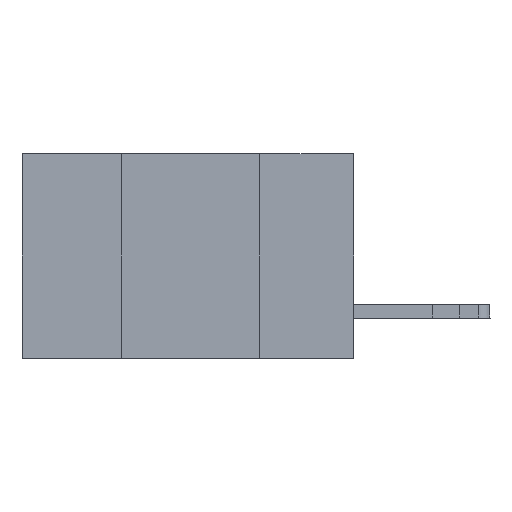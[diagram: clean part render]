
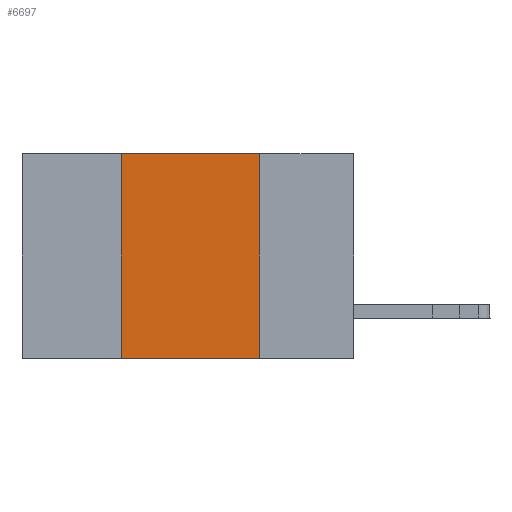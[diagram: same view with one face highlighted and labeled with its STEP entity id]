
A CAD part, left-side view. The second image highlights one B-rep face of the part: STEP entity #6697.
In plain terms, the highlighted planar face has unit normal (-1, 0, 0).
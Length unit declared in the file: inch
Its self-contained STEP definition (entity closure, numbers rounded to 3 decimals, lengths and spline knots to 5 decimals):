
#640 = PLANE ( 'NONE',  #17422 ) ;
#1142 = VERTEX_POINT ( 'NONE', #27740 ) ;
#1392 = LINE ( 'NONE', #13812, #27585 ) ;
#4769 = CARTESIAN_POINT ( 'NONE',  ( 0., 0.6, 0. ) ) ;
#6697 = ADVANCED_FACE ( 'NONE', ( #7841 ), #640, .F. ) ;
#7841 = FACE_OUTER_BOUND ( 'NONE', #24809, .T. ) ;
#8681 = EDGE_CURVE ( 'NONE', #14372, #1142, #14661, .T. ) ;
#9336 = CARTESIAN_POINT ( 'NONE',  ( 0., 0.17, 0. ) ) ;
#9477 = ORIENTED_EDGE ( 'NONE', *, *, #16613, .F. ) ;
#11644 = LINE ( 'NONE', #9336, #30288 ) ;
#12538 = EDGE_CURVE ( 'NONE', #13176, #19189, #24336, .T. ) ;
#13176 = VERTEX_POINT ( 'NONE', #31126 ) ;
#13812 = CARTESIAN_POINT ( 'NONE',  ( 0., 0.42, 0. ) ) ;
#14372 = VERTEX_POINT ( 'NONE', #31003 ) ;
#14661 = LINE ( 'NONE', #17255, #20536 ) ;
#16576 = DIRECTION ( 'NONE',  ( 0., 0., 1. ) ) ;
#16613 = EDGE_CURVE ( 'NONE', #14372, #13176, #1392, .T. ) ;
#16631 = CARTESIAN_POINT ( 'NONE',  ( 0., 0.17, 0. ) ) ;
#16641 = ORIENTED_EDGE ( 'NONE', *, *, #12538, .F. ) ;
#16780 = DIRECTION ( 'NONE',  ( 0., -1., 0. ) ) ;
#17255 = CARTESIAN_POINT ( 'NONE',  ( 0., 0.6, -0.37 ) ) ;
#17422 = AXIS2_PLACEMENT_3D ( 'NONE', #25146, #27576, #25773 ) ;
#17543 = ORIENTED_EDGE ( 'NONE', *, *, #18163, .F. ) ;
#17739 = ORIENTED_EDGE ( 'NONE', *, *, #8681, .T. ) ;
#18111 = VECTOR ( 'NONE', #22364, 39.37008 ) ;
#18163 = EDGE_CURVE ( 'NONE', #19189, #1142, #11644, .T. ) ;
#19189 = VERTEX_POINT ( 'NONE', #16631 ) ;
#20536 = VECTOR ( 'NONE', #16780, 39.37008 ) ;
#21564 = DIRECTION ( 'NONE',  ( 0., 0., -1. ) ) ;
#22364 = DIRECTION ( 'NONE',  ( 0., -1., 0. ) ) ;
#24336 = LINE ( 'NONE', #4769, #18111 ) ;
#24809 = EDGE_LOOP ( 'NONE', ( #17543, #16641, #9477, #17739 ) ) ;
#25146 = CARTESIAN_POINT ( 'NONE',  ( 0., 0.6, 0. ) ) ;
#25773 = DIRECTION ( 'NONE',  ( 0., 0., -1. ) ) ;
#27576 = DIRECTION ( 'NONE',  ( 1., 0., 0. ) ) ;
#27585 = VECTOR ( 'NONE', #16576, 39.37008 ) ;
#27740 = CARTESIAN_POINT ( 'NONE',  ( 0., 0.17, -0.37 ) ) ;
#30288 = VECTOR ( 'NONE', #21564, 39.37008 ) ;
#31003 = CARTESIAN_POINT ( 'NONE',  ( 0., 0.42, -0.37 ) ) ;
#31126 = CARTESIAN_POINT ( 'NONE',  ( 0., 0.42, 0. ) ) ;
